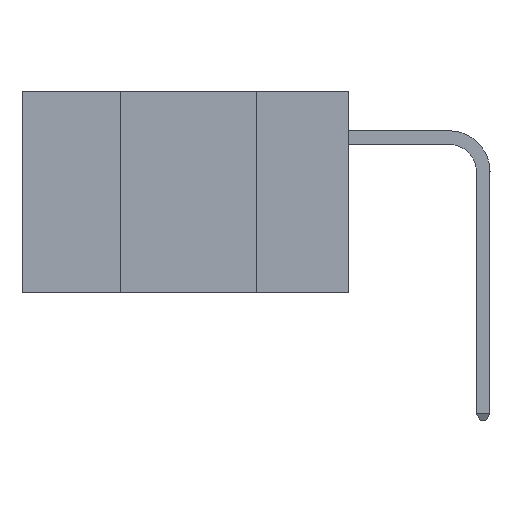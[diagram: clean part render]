
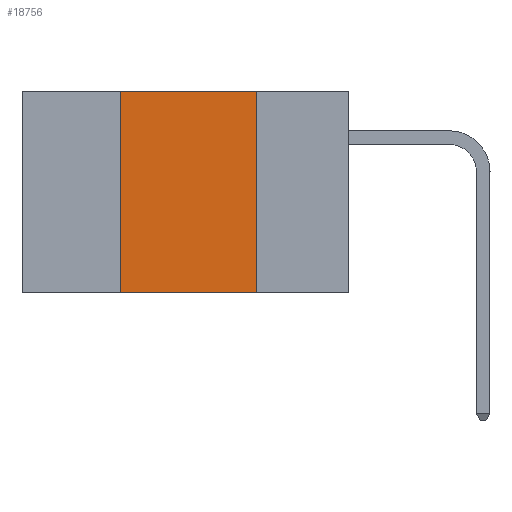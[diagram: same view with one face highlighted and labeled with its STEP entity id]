
A CAD part, left-side view. The second image highlights one B-rep face of the part: STEP entity #18756.
In plain terms, the highlighted planar face has unit normal (-1, 0, 0).
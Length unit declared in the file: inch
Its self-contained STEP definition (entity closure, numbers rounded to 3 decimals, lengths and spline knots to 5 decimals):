
#658 = LINE ( 'NONE', #2813, #1239 ) ;
#780 = VECTOR ( 'NONE', #27988, 39.37008 ) ;
#1239 = VECTOR ( 'NONE', #6338, 39.37008 ) ;
#2813 = CARTESIAN_POINT ( 'NONE',  ( 0., 0.42, 0. ) ) ;
#5137 = ORIENTED_EDGE ( 'NONE', *, *, #23228, .F. ) ;
#6338 = DIRECTION ( 'NONE',  ( 0., 0., 1. ) ) ;
#6895 = CARTESIAN_POINT ( 'NONE',  ( 0., 0.6, -0.37 ) ) ;
#7499 = CARTESIAN_POINT ( 'NONE',  ( 0., 0.17, 0. ) ) ;
#9116 = CARTESIAN_POINT ( 'NONE',  ( 0., 0.6, 0. ) ) ;
#9169 = CARTESIAN_POINT ( 'NONE',  ( 0., 0.17, 0. ) ) ;
#9286 = VECTOR ( 'NONE', #12218, 39.37008 ) ;
#9531 = ORIENTED_EDGE ( 'NONE', *, *, #10214, .F. ) ;
#10214 = EDGE_CURVE ( 'NONE', #42476, #33262, #24085, .T. ) ;
#12218 = DIRECTION ( 'NONE',  ( 0., -1., 0. ) ) ;
#12995 = FACE_OUTER_BOUND ( 'NONE', #32301, .T. ) ;
#16996 = PLANE ( 'NONE',  #20467 ) ;
#17906 = VERTEX_POINT ( 'NONE', #29678 ) ;
#18756 = ADVANCED_FACE ( 'NONE', ( #12995 ), #16996, .F. ) ;
#20190 = EDGE_CURVE ( 'NONE', #33262, #27021, #26038, .T. ) ;
#20467 = AXIS2_PLACEMENT_3D ( 'NONE', #27656, #20496, #24027 ) ;
#20496 = DIRECTION ( 'NONE',  ( 1., 0., 0. ) ) ;
#23228 = EDGE_CURVE ( 'NONE', #17906, #42476, #658, .T. ) ;
#24027 = DIRECTION ( 'NONE',  ( 0., 0., -1. ) ) ;
#24085 = LINE ( 'NONE', #9116, #9286 ) ;
#26038 = LINE ( 'NONE', #7499, #780 ) ;
#27021 = VERTEX_POINT ( 'NONE', #30720 ) ;
#27656 = CARTESIAN_POINT ( 'NONE',  ( 0., 0.6, 0. ) ) ;
#27988 = DIRECTION ( 'NONE',  ( 0., 0., -1. ) ) ;
#28591 = EDGE_CURVE ( 'NONE', #17906, #27021, #44661, .T. ) ;
#29297 = VECTOR ( 'NONE', #35183, 39.37008 ) ;
#29678 = CARTESIAN_POINT ( 'NONE',  ( 0., 0.42, -0.37 ) ) ;
#30720 = CARTESIAN_POINT ( 'NONE',  ( 0., 0.17, -0.37 ) ) ;
#32301 = EDGE_LOOP ( 'NONE', ( #38929, #9531, #5137, #41145 ) ) ;
#33262 = VERTEX_POINT ( 'NONE', #9169 ) ;
#35183 = DIRECTION ( 'NONE',  ( 0., -1., 0. ) ) ;
#38929 = ORIENTED_EDGE ( 'NONE', *, *, #20190, .F. ) ;
#41145 = ORIENTED_EDGE ( 'NONE', *, *, #28591, .T. ) ;
#42464 = CARTESIAN_POINT ( 'NONE',  ( 0., 0.42, 0. ) ) ;
#42476 = VERTEX_POINT ( 'NONE', #42464 ) ;
#44661 = LINE ( 'NONE', #6895, #29297 ) ;
